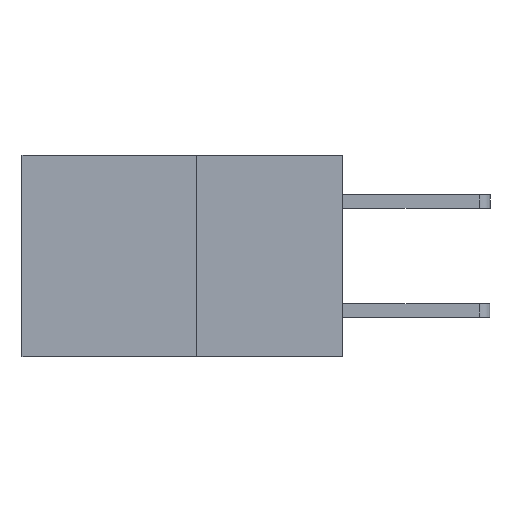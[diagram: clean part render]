
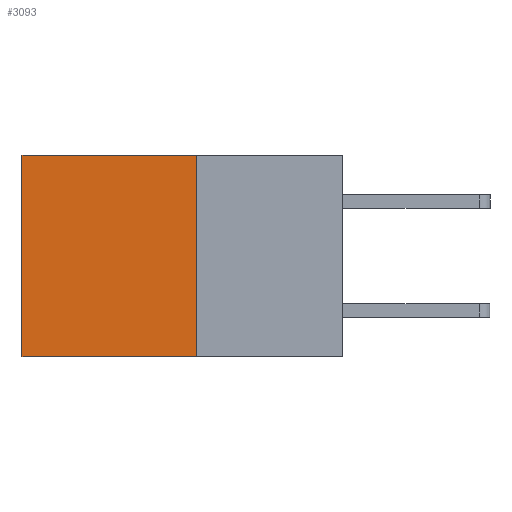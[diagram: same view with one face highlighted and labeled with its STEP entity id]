
A CAD part, left-side view. The second image highlights one B-rep face of the part: STEP entity #3093.
In plain terms, the highlighted planar face has unit normal (-1, 0, 0).
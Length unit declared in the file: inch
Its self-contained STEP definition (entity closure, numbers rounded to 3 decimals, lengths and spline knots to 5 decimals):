
#15 = EDGE_CURVE ( 'NONE', #1164, #1472, #1451, .T. ) ;
#42 = ORIENTED_EDGE ( 'NONE', *, *, #15, .F. ) ;
#60 = ORIENTED_EDGE ( 'NONE', *, *, #2895, .F. ) ;
#146 = VERTEX_POINT ( 'NONE', #4344 ) ;
#392 = VECTOR ( 'NONE', #1424, 39.37008 ) ;
#434 = DIRECTION ( 'NONE',  ( 1., 0., 0. ) ) ;
#600 = DIRECTION ( 'NONE',  ( 0., 1., 0. ) ) ;
#749 = AXIS2_PLACEMENT_3D ( 'NONE', #5500, #434, #2726 ) ;
#1164 = VERTEX_POINT ( 'NONE', #3372 ) ;
#1209 = EDGE_CURVE ( 'NONE', #1164, #6046, #4253, .T. ) ;
#1299 = CARTESIAN_POINT ( 'NONE',  ( 0.277, 0.59, 0. ) ) ;
#1424 = DIRECTION ( 'NONE',  ( 0., 0., -1. ) ) ;
#1451 = LINE ( 'NONE', #4800, #4720 ) ;
#1472 = VERTEX_POINT ( 'NONE', #6522 ) ;
#1964 = LINE ( 'NONE', #2681, #392 ) ;
#2038 = CARTESIAN_POINT ( 'NONE',  ( 0.277, 0.27, 0. ) ) ;
#2681 = CARTESIAN_POINT ( 'NONE',  ( 0.277, 0.59, -0.37 ) ) ;
#2726 = DIRECTION ( 'NONE',  ( 0., 0., -1. ) ) ;
#2895 = EDGE_CURVE ( 'NONE', #1472, #146, #6562, .T. ) ;
#3093 = ADVANCED_FACE ( 'NONE', ( #3123 ), #6707, .F. ) ;
#3123 = FACE_OUTER_BOUND ( 'NONE', #7753, .T. ) ;
#3372 = CARTESIAN_POINT ( 'NONE',  ( 0.277, 0.27, 0. ) ) ;
#3654 = DIRECTION ( 'NONE',  ( 0., 1., 0. ) ) ;
#3837 = EDGE_CURVE ( 'NONE', #6046, #146, #1964, .T. ) ;
#4061 = VECTOR ( 'NONE', #3654, 39.37008 ) ;
#4182 = CARTESIAN_POINT ( 'NONE',  ( 0.277, 0.27, -0.37 ) ) ;
#4253 = LINE ( 'NONE', #2038, #4061 ) ;
#4344 = CARTESIAN_POINT ( 'NONE',  ( 0.277, 0.59, -0.37 ) ) ;
#4720 = VECTOR ( 'NONE', #7268, 39.37008 ) ;
#4800 = CARTESIAN_POINT ( 'NONE',  ( 0.277, 0.27, -0.37 ) ) ;
#5500 = CARTESIAN_POINT ( 'NONE',  ( 0.277, 0.27, -0.37 ) ) ;
#5582 = ORIENTED_EDGE ( 'NONE', *, *, #3837, .T. ) ;
#6046 = VERTEX_POINT ( 'NONE', #1299 ) ;
#6396 = VECTOR ( 'NONE', #600, 39.37008 ) ;
#6522 = CARTESIAN_POINT ( 'NONE',  ( 0.277, 0.27, -0.37 ) ) ;
#6562 = LINE ( 'NONE', #4182, #6396 ) ;
#6707 = PLANE ( 'NONE',  #749 ) ;
#6907 = ORIENTED_EDGE ( 'NONE', *, *, #1209, .T. ) ;
#7268 = DIRECTION ( 'NONE',  ( 0., 0., -1. ) ) ;
#7753 = EDGE_LOOP ( 'NONE', ( #5582, #60, #42, #6907 ) ) ;
